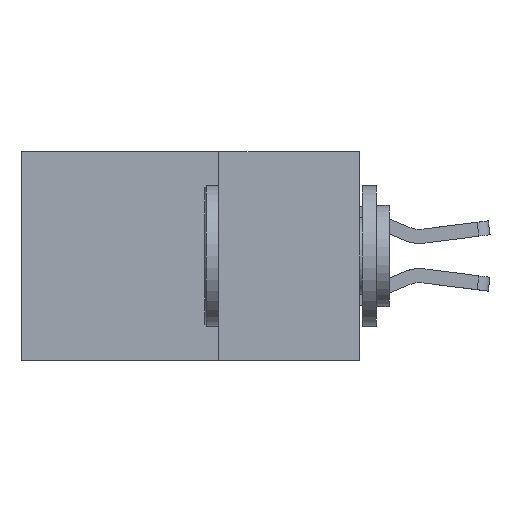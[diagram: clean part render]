
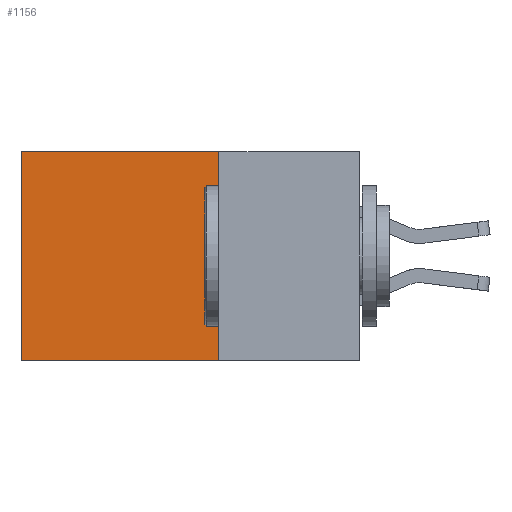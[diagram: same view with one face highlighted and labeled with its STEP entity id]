
A CAD part, left-side view. The second image highlights one B-rep face of the part: STEP entity #1156.
In plain terms, the highlighted planar face has unit normal (-1, 0, 0).
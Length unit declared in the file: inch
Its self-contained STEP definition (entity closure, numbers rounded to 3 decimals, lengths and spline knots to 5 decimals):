
#238 = LINE ( 'NONE', #976, #13048 ) ;
#242 = EDGE_CURVE ( 'NONE', #4535, #11901, #869, .T. ) ;
#866 = DIRECTION ( 'NONE',  ( 0., 1., 0. ) ) ;
#869 = LINE ( 'NONE', #2888, #11724 ) ;
#976 = CARTESIAN_POINT ( 'NONE',  ( 0.2875, 0.6, 0. ) ) ;
#994 = CARTESIAN_POINT ( 'NONE',  ( 0.2875, 0.25, -0.37 ) ) ;
#1156 = ADVANCED_FACE ( 'NONE', ( #9567 ), #4704, .F. ) ;
#1479 = VERTEX_POINT ( 'NONE', #4600 ) ;
#2061 = DIRECTION ( 'NONE',  ( 0., 0., -1. ) ) ;
#2313 = EDGE_LOOP ( 'NONE', ( #6240, #6311, #6405, #6432 ) ) ;
#2519 = DIRECTION ( 'NONE',  ( 0., 0., -1. ) ) ;
#2888 = CARTESIAN_POINT ( 'NONE',  ( 0.2875, 0.25, 0. ) ) ;
#3110 = AXIS2_PLACEMENT_3D ( 'NONE', #4689, #12277, #2519 ) ;
#4134 = CARTESIAN_POINT ( 'NONE',  ( 0.2875, 0.25, 0. ) ) ;
#4345 = LINE ( 'NONE', #994, #9599 ) ;
#4535 = VERTEX_POINT ( 'NONE', #7417 ) ;
#4600 = CARTESIAN_POINT ( 'NONE',  ( 0.2875, 0.25, -0.37 ) ) ;
#4689 = CARTESIAN_POINT ( 'NONE',  ( 0.2875, 0.25, 0. ) ) ;
#4704 = PLANE ( 'NONE',  #3110 ) ;
#4755 = CARTESIAN_POINT ( 'NONE',  ( 0.2875, 0.6, 0. ) ) ;
#4945 = DIRECTION ( 'NONE',  ( 0., 1., 0. ) ) ;
#5087 = DIRECTION ( 'NONE',  ( 0., 0., -1. ) ) ;
#5686 = VERTEX_POINT ( 'NONE', #12694 ) ;
#5901 = EDGE_CURVE ( 'NONE', #1479, #5686, #4345, .T. ) ;
#6240 = ORIENTED_EDGE ( 'NONE', *, *, #11199, .T. ) ;
#6311 = ORIENTED_EDGE ( 'NONE', *, *, #5901, .F. ) ;
#6405 = ORIENTED_EDGE ( 'NONE', *, *, #6962, .F. ) ;
#6432 = ORIENTED_EDGE ( 'NONE', *, *, #242, .T. ) ;
#6962 = EDGE_CURVE ( 'NONE', #4535, #1479, #8247, .T. ) ;
#7417 = CARTESIAN_POINT ( 'NONE',  ( 0.2875, 0.25, 0. ) ) ;
#8247 = LINE ( 'NONE', #4134, #13090 ) ;
#9567 = FACE_OUTER_BOUND ( 'NONE', #2313, .T. ) ;
#9599 = VECTOR ( 'NONE', #4945, 39.37008 ) ;
#11199 = EDGE_CURVE ( 'NONE', #11901, #5686, #238, .T. ) ;
#11724 = VECTOR ( 'NONE', #866, 39.37008 ) ;
#11901 = VERTEX_POINT ( 'NONE', #4755 ) ;
#12277 = DIRECTION ( 'NONE',  ( 1., 0., 0. ) ) ;
#12694 = CARTESIAN_POINT ( 'NONE',  ( 0.2875, 0.6, -0.37 ) ) ;
#13048 = VECTOR ( 'NONE', #2061, 39.37008 ) ;
#13090 = VECTOR ( 'NONE', #5087, 39.37008 ) ;
